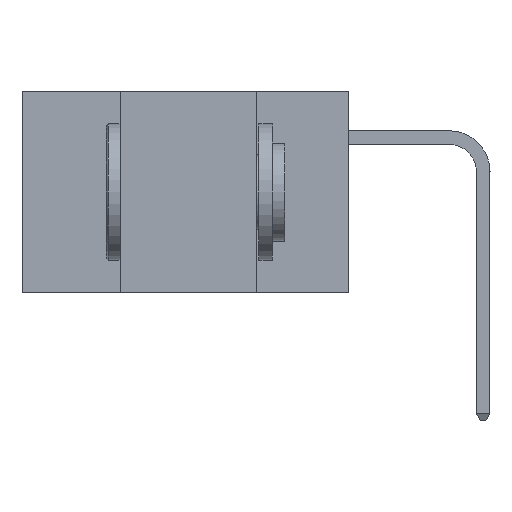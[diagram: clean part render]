
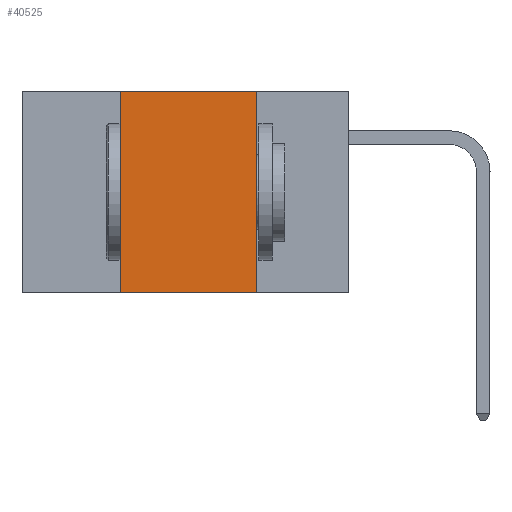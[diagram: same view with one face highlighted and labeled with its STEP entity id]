
A CAD part, left-side view. The second image highlights one B-rep face of the part: STEP entity #40525.
In plain terms, the highlighted planar face has unit normal (-1, 0, 0).
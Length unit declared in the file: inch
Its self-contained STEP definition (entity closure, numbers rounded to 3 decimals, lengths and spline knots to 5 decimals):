
#848 = CARTESIAN_POINT ( 'NONE',  ( 0., 0.42, 0. ) ) ;
#1044 = DIRECTION ( 'NONE',  ( 0., -1., 0. ) ) ;
#2989 = EDGE_CURVE ( 'NONE', #23038, #38930, #4308, .T. ) ;
#4014 = CARTESIAN_POINT ( 'NONE',  ( 0., 0.17, -0.37 ) ) ;
#4105 = DIRECTION ( 'NONE',  ( 0., 0., 1. ) ) ;
#4272 = DIRECTION ( 'NONE',  ( 0., 0., -1. ) ) ;
#4308 = LINE ( 'NONE', #30379, #36498 ) ;
#6326 = VECTOR ( 'NONE', #4105, 39.37008 ) ;
#6905 = VERTEX_POINT ( 'NONE', #27803 ) ;
#8400 = FACE_OUTER_BOUND ( 'NONE', #19607, .T. ) ;
#10320 = PLANE ( 'NONE',  #20632 ) ;
#11808 = DIRECTION ( 'NONE',  ( 0., -1., 0. ) ) ;
#11870 = LINE ( 'NONE', #12135, #25377 ) ;
#12135 = CARTESIAN_POINT ( 'NONE',  ( 0., 0.17, 0. ) ) ;
#12138 = EDGE_CURVE ( 'NONE', #27626, #6905, #12624, .T. ) ;
#12241 = ORIENTED_EDGE ( 'NONE', *, *, #12138, .F. ) ;
#12624 = LINE ( 'NONE', #23032, #36497 ) ;
#12728 = EDGE_CURVE ( 'NONE', #23038, #27626, #14611, .T. ) ;
#14611 = LINE ( 'NONE', #848, #6326 ) ;
#14970 = CARTESIAN_POINT ( 'NONE',  ( 0., 0.42, -0.37 ) ) ;
#19607 = EDGE_LOOP ( 'NONE', ( #35595, #12241, #39030, #38561 ) ) ;
#20632 = AXIS2_PLACEMENT_3D ( 'NONE', #38462, #22885, #4272 ) ;
#22885 = DIRECTION ( 'NONE',  ( 1., 0., 0. ) ) ;
#23032 = CARTESIAN_POINT ( 'NONE',  ( 0., 0.6, 0. ) ) ;
#23038 = VERTEX_POINT ( 'NONE', #14970 ) ;
#24389 = EDGE_CURVE ( 'NONE', #6905, #38930, #11870, .T. ) ;
#25377 = VECTOR ( 'NONE', #37027, 39.37008 ) ;
#27626 = VERTEX_POINT ( 'NONE', #29547 ) ;
#27803 = CARTESIAN_POINT ( 'NONE',  ( 0., 0.17, 0. ) ) ;
#29547 = CARTESIAN_POINT ( 'NONE',  ( 0., 0.42, 0. ) ) ;
#30379 = CARTESIAN_POINT ( 'NONE',  ( 0., 0.6, -0.37 ) ) ;
#35595 = ORIENTED_EDGE ( 'NONE', *, *, #24389, .F. ) ;
#36497 = VECTOR ( 'NONE', #1044, 39.37008 ) ;
#36498 = VECTOR ( 'NONE', #11808, 39.37008 ) ;
#37027 = DIRECTION ( 'NONE',  ( 0., 0., -1. ) ) ;
#38462 = CARTESIAN_POINT ( 'NONE',  ( 0., 0.6, 0. ) ) ;
#38561 = ORIENTED_EDGE ( 'NONE', *, *, #2989, .T. ) ;
#38930 = VERTEX_POINT ( 'NONE', #4014 ) ;
#39030 = ORIENTED_EDGE ( 'NONE', *, *, #12728, .F. ) ;
#40525 = ADVANCED_FACE ( 'NONE', ( #8400 ), #10320, .F. ) ;
